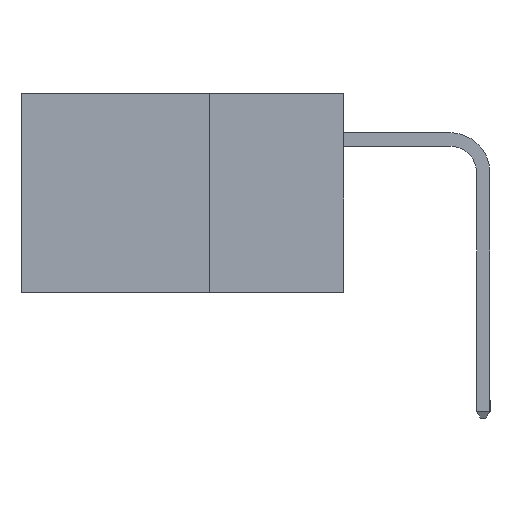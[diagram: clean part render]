
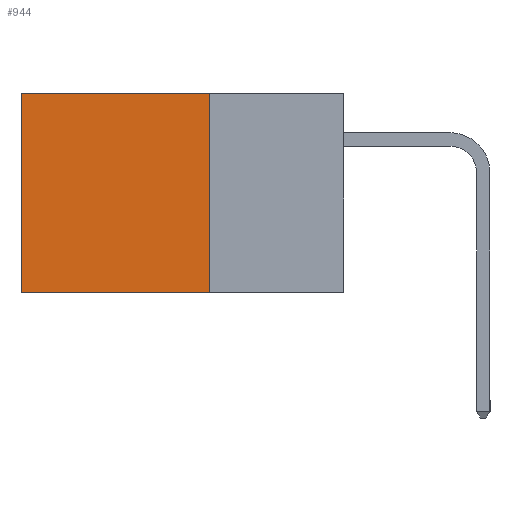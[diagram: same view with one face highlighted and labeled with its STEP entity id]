
A CAD part, left-side view. The second image highlights one B-rep face of the part: STEP entity #944.
In plain terms, the highlighted planar face has unit normal (-1, 0, 0).
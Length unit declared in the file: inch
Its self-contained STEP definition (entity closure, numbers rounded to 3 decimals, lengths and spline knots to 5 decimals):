
#30 = CARTESIAN_POINT ( 'NONE',  ( 0.2615, 0.6, -0.37 ) ) ;
#497 = CARTESIAN_POINT ( 'NONE',  ( 0.2615, 0.6, -0.37 ) ) ;
#682 = CARTESIAN_POINT ( 'NONE',  ( 0.2615, 0.25, -0.37 ) ) ;
#836 = PLANE ( 'NONE',  #4604 ) ;
#944 = ADVANCED_FACE ( 'NONE', ( #4383 ), #836, .F. ) ;
#963 = DIRECTION ( 'NONE',  ( 0., 0., -1. ) ) ;
#990 = DIRECTION ( 'NONE',  ( 1., 0., 0. ) ) ;
#1353 = CARTESIAN_POINT ( 'NONE',  ( 0.2615, 0.25, -0.37 ) ) ;
#1377 = VERTEX_POINT ( 'NONE', #8143 ) ;
#1655 = VERTEX_POINT ( 'NONE', #1353 ) ;
#1747 = EDGE_LOOP ( 'NONE', ( #5096, #5191, #2423, #1762 ) ) ;
#1762 = ORIENTED_EDGE ( 'NONE', *, *, #5404, .T. ) ;
#2301 = VERTEX_POINT ( 'NONE', #8351 ) ;
#2423 = ORIENTED_EDGE ( 'NONE', *, *, #10246, .F. ) ;
#2804 = LINE ( 'NONE', #497, #9543 ) ;
#2861 = CARTESIAN_POINT ( 'NONE',  ( 0.2615, 0.25, -0.37 ) ) ;
#3641 = LINE ( 'NONE', #4533, #8405 ) ;
#4354 = VERTEX_POINT ( 'NONE', #30 ) ;
#4383 = FACE_OUTER_BOUND ( 'NONE', #1747, .T. ) ;
#4533 = CARTESIAN_POINT ( 'NONE',  ( 0.2615, 0.25, -0.37 ) ) ;
#4604 = AXIS2_PLACEMENT_3D ( 'NONE', #682, #990, #963 ) ;
#5038 = LINE ( 'NONE', #2861, #9159 ) ;
#5096 = ORIENTED_EDGE ( 'NONE', *, *, #9292, .T. ) ;
#5191 = ORIENTED_EDGE ( 'NONE', *, *, #6887, .F. ) ;
#5404 = EDGE_CURVE ( 'NONE', #2301, #1377, #5887, .T. ) ;
#5829 = CARTESIAN_POINT ( 'NONE',  ( 0.2615, 0.25, 0. ) ) ;
#5887 = LINE ( 'NONE', #5829, #7812 ) ;
#5903 = DIRECTION ( 'NONE',  ( 0., 0., -1. ) ) ;
#6654 = DIRECTION ( 'NONE',  ( 0., 1., 0. ) ) ;
#6887 = EDGE_CURVE ( 'NONE', #1655, #4354, #3641, .T. ) ;
#7170 = DIRECTION ( 'NONE',  ( 0., 0., -1. ) ) ;
#7812 = VECTOR ( 'NONE', #6654, 39.37008 ) ;
#8143 = CARTESIAN_POINT ( 'NONE',  ( 0.2615, 0.6, 0. ) ) ;
#8351 = CARTESIAN_POINT ( 'NONE',  ( 0.2615, 0.25, 0. ) ) ;
#8405 = VECTOR ( 'NONE', #10270, 39.37008 ) ;
#9159 = VECTOR ( 'NONE', #7170, 39.37008 ) ;
#9292 = EDGE_CURVE ( 'NONE', #1377, #4354, #2804, .T. ) ;
#9543 = VECTOR ( 'NONE', #5903, 39.37008 ) ;
#10246 = EDGE_CURVE ( 'NONE', #2301, #1655, #5038, .T. ) ;
#10270 = DIRECTION ( 'NONE',  ( 0., 1., 0. ) ) ;
